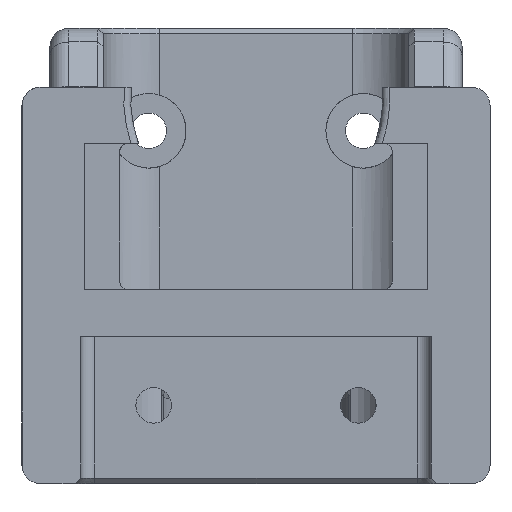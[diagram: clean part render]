
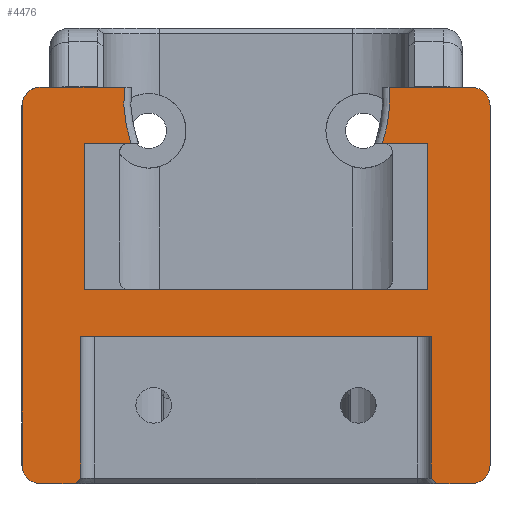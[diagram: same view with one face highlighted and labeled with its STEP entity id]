
A CAD part, front view. The second image highlights one B-rep face of the part: STEP entity #4476.
In plain terms, the highlighted planar face has unit normal (0, -1, 0).
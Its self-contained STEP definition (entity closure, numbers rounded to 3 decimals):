
#76=ELLIPSE('',#4882,2.,2.);
#77=ELLIPSE('',#4885,2.,2.);
#150=PLANE('',#4881);
#224=LINE('',#6659,#567);
#228=LINE('',#6671,#571);
#399=LINE('',#8443,#742);
#424=LINE('',#8539,#767);
#440=LINE('',#8845,#783);
#442=LINE('',#8940,#785);
#446=LINE('',#8950,#789);
#447=LINE('',#8953,#790);
#448=LINE('',#8955,#791);
#449=LINE('',#8957,#792);
#450=LINE('',#8959,#793);
#451=LINE('',#8960,#794);
#452=LINE('',#8964,#795);
#453=LINE('',#8968,#796);
#454=LINE('',#8970,#797);
#455=LINE('',#8971,#798);
#567=VECTOR('',#5177,10.);
#571=VECTOR('',#5185,10.);
#742=VECTOR('',#5724,10.);
#767=VECTOR('',#5797,10.);
#783=VECTOR('',#5869,10.);
#785=VECTOR('',#5881,10.);
#789=VECTOR('',#5889,10.);
#790=VECTOR('',#5892,10.);
#791=VECTOR('',#5893,10.);
#792=VECTOR('',#5894,10.);
#793=VECTOR('',#5895,10.);
#794=VECTOR('',#5896,10.);
#795=VECTOR('',#5899,10.);
#796=VECTOR('',#5904,10.);
#797=VECTOR('',#5905,10.);
#798=VECTOR('',#5906,10.);
#1164=FACE_OUTER_BOUND('',#1435,.T.);
#1435=EDGE_LOOP('',(#3844,#3845,#3846,#3847,#3848,#3849,#3850,#3851,#3852,
#3853,#3854,#3855,#3856,#3857,#3858,#3859,#3860,#3861,#3862,#3863,#3864,
#3865));
#1669=CIRCLE('',#4879,14.25);
#1670=CIRCLE('',#4883,2.);
#1671=CIRCLE('',#4884,2.);
#1672=CIRCLE('',#4886,14.25);
#1892=VERTEX_POINT('',#6656);
#1893=VERTEX_POINT('',#6658);
#1898=VERTEX_POINT('',#6668);
#1899=VERTEX_POINT('',#6670);
#2113=VERTEX_POINT('',#8440);
#2114=VERTEX_POINT('',#8442);
#2134=VERTEX_POINT('',#8527);
#2135=VERTEX_POINT('',#8538);
#2167=VERTEX_POINT('',#8842);
#2168=VERTEX_POINT('',#8844);
#2171=VERTEX_POINT('',#8926);
#2172=VERTEX_POINT('',#8939);
#2175=VERTEX_POINT('',#8947);
#2176=VERTEX_POINT('',#8949);
#2177=VERTEX_POINT('',#8952);
#2178=VERTEX_POINT('',#8954);
#2179=VERTEX_POINT('',#8956);
#2180=VERTEX_POINT('',#8958);
#2181=VERTEX_POINT('',#8961);
#2182=VERTEX_POINT('',#8963);
#2183=VERTEX_POINT('',#8967);
#2184=VERTEX_POINT('',#8969);
#2329=EDGE_CURVE('',#1892,#1893,#224,.T.);
#2335=EDGE_CURVE('',#1898,#1899,#228,.T.);
#2673=EDGE_CURVE('',#2114,#2113,#399,.T.);
#2710=EDGE_CURVE('',#2134,#2135,#424,.T.);
#2757=EDGE_CURVE('',#2167,#2168,#440,.T.);
#2763=EDGE_CURVE('',#2114,#2171,#1669,.T.);
#2765=EDGE_CURVE('',#2171,#2172,#442,.T.);
#2769=EDGE_CURVE('',#2175,#2113,#76,.T.);
#2770=EDGE_CURVE('',#2176,#2175,#446,.T.);
#2771=EDGE_CURVE('',#1899,#2176,#1670,.T.);
#2772=EDGE_CURVE('',#2177,#1898,#447,.T.);
#2773=EDGE_CURVE('',#2177,#2178,#448,.T.);
#2774=EDGE_CURVE('',#2178,#2179,#449,.T.);
#2775=EDGE_CURVE('',#2180,#2179,#450,.T.);
#2776=EDGE_CURVE('',#1893,#2180,#451,.T.);
#2777=EDGE_CURVE('',#2181,#1892,#1671,.T.);
#2778=EDGE_CURVE('',#2181,#2182,#452,.T.);
#2779=EDGE_CURVE('',#2135,#2182,#77,.T.);
#2780=EDGE_CURVE('',#2168,#2134,#1672,.T.);
#2781=EDGE_CURVE('',#2167,#2183,#453,.T.);
#2782=EDGE_CURVE('',#2183,#2184,#454,.T.);
#2783=EDGE_CURVE('',#2184,#2172,#455,.T.);
#3844=ORIENTED_EDGE('',*,*,#2763,.F.);
#3845=ORIENTED_EDGE('',*,*,#2673,.T.);
#3846=ORIENTED_EDGE('',*,*,#2769,.F.);
#3847=ORIENTED_EDGE('',*,*,#2770,.F.);
#3848=ORIENTED_EDGE('',*,*,#2771,.F.);
#3849=ORIENTED_EDGE('',*,*,#2335,.F.);
#3850=ORIENTED_EDGE('',*,*,#2772,.F.);
#3851=ORIENTED_EDGE('',*,*,#2773,.T.);
#3852=ORIENTED_EDGE('',*,*,#2774,.T.);
#3853=ORIENTED_EDGE('',*,*,#2775,.F.);
#3854=ORIENTED_EDGE('',*,*,#2776,.F.);
#3855=ORIENTED_EDGE('',*,*,#2329,.F.);
#3856=ORIENTED_EDGE('',*,*,#2777,.F.);
#3857=ORIENTED_EDGE('',*,*,#2778,.T.);
#3858=ORIENTED_EDGE('',*,*,#2779,.F.);
#3859=ORIENTED_EDGE('',*,*,#2710,.F.);
#3860=ORIENTED_EDGE('',*,*,#2780,.F.);
#3861=ORIENTED_EDGE('',*,*,#2757,.F.);
#3862=ORIENTED_EDGE('',*,*,#2781,.T.);
#3863=ORIENTED_EDGE('',*,*,#2782,.T.);
#3864=ORIENTED_EDGE('',*,*,#2783,.T.);
#3865=ORIENTED_EDGE('',*,*,#2765,.F.);
#4476=ADVANCED_FACE('',(#1164),#150,.T.);
#4879=AXIS2_PLACEMENT_3D('',#8927,#5877,#5878);
#4881=AXIS2_PLACEMENT_3D('',#8946,#5885,#5886);
#4882=AXIS2_PLACEMENT_3D('',#8948,#5887,#5888);
#4883=AXIS2_PLACEMENT_3D('',#8951,#5890,#5891);
#4884=AXIS2_PLACEMENT_3D('',#8962,#5897,#5898);
#4885=AXIS2_PLACEMENT_3D('',#8965,#5900,#5901);
#4886=AXIS2_PLACEMENT_3D('',#8966,#5902,#5903);
#5177=DIRECTION('',(-1.,0.,0.));
#5185=DIRECTION('',(-1.,0.,0.));
#5724=DIRECTION('',(-1.,0.,0.));
#5797=DIRECTION('',(1.,0.,0.));
#5869=DIRECTION('',(-1.,0.,0.));
#5877=DIRECTION('center_axis',(0.,-1.,0.));
#5878=DIRECTION('ref_axis',(-0.992,0.,-0.127));
#5881=DIRECTION('',(-1.,0.,0.));
#5885=DIRECTION('center_axis',(0.,-1.,0.));
#5886=DIRECTION('ref_axis',(1.,0.,0.));
#5887=DIRECTION('center_axis',(0.,1.,0.));
#5888=DIRECTION('ref_axis',(0.,0.,1.));
#5889=DIRECTION('',(0.,0.,1.));
#5890=DIRECTION('center_axis',(0.,1.,0.));
#5891=DIRECTION('ref_axis',(-0.707,0.,-0.707));
#5892=DIRECTION('',(-0.707,0.,-0.707));
#5893=DIRECTION('',(0.,0.,1.));
#5894=DIRECTION('',(1.,0.,0.));
#5895=DIRECTION('',(0.,0.,1.));
#5896=DIRECTION('',(-0.707,0.,0.707));
#5897=DIRECTION('center_axis',(0.,1.,0.));
#5898=DIRECTION('ref_axis',(0.707,0.,-0.707));
#5899=DIRECTION('',(0.,0.,1.));
#5900=DIRECTION('center_axis',(0.,1.,0.));
#5901=DIRECTION('ref_axis',(0.,0.,1.));
#5902=DIRECTION('center_axis',(0.,-1.,0.));
#5903=DIRECTION('ref_axis',(0.992,0.,-0.127));
#5904=DIRECTION('',(0.,0.,-1.));
#5905=DIRECTION('',(-1.,0.,0.));
#5906=DIRECTION('',(0.,0.,1.));
#6656=CARTESIAN_POINT('',(39.053,-26.,-157.388));
#6658=CARTESIAN_POINT('',(35.353,-26.,-157.388));
#6659=CARTESIAN_POINT('',(26.915,-26.,-157.388));
#6668=CARTESIAN_POINT('',(-3.4,-26.,-157.388));
#6670=CARTESIAN_POINT('',(-7.1,-26.,-157.388));
#6671=CARTESIAN_POINT('',(26.915,-26.,-157.388));
#8440=CARTESIAN_POINT('',(-7.1,-26.,-114.899));
#8442=CARTESIAN_POINT('',(1.865,-26.,-114.899));
#8443=CARTESIAN_POINT('',(-5.325,-26.,-114.899));
#8527=CARTESIAN_POINT('',(30.24,-26.,-114.899));
#8538=CARTESIAN_POINT('',(39.053,-26.,-114.899));
#8539=CARTESIAN_POINT('',(37.278,-26.,-114.899));
#8842=CARTESIAN_POINT('',(34.353,-26.,-120.899));
#8844=CARTESIAN_POINT('',(29.517,-26.,-120.899));
#8845=CARTESIAN_POINT('',(26.84,-26.,-120.899));
#8926=CARTESIAN_POINT('',(2.588,-26.,-120.899));
#8927=CARTESIAN_POINT('Origin',(16.053,-26.,-116.233));
#8939=CARTESIAN_POINT('',(-2.4,-26.,-120.899));
#8940=CARTESIAN_POINT('',(26.84,-26.,-120.899));
#8946=CARTESIAN_POINT('Origin',(-5.9,-26.,-136.589));
#8947=CARTESIAN_POINT('',(-9.1,-26.,-116.899));
#8948=CARTESIAN_POINT('Origin',(-7.1,-26.,-116.899));
#8949=CARTESIAN_POINT('',(-9.1,-26.,-155.388));
#8950=CARTESIAN_POINT('',(-9.1,-26.,-157.388));
#8951=CARTESIAN_POINT('Origin',(-7.1,-26.,-155.388));
#8952=CARTESIAN_POINT('',(-2.8,-26.,-156.788));
#8953=CARTESIAN_POINT('',(1.325,-26.,-152.663));
#8954=CARTESIAN_POINT('',(-2.8,-26.,-141.588));
#8955=CARTESIAN_POINT('',(-2.8,-26.,-143.888));
#8956=CARTESIAN_POINT('',(34.753,-26.,-141.588));
#8957=CARTESIAN_POINT('',(-4.5,-26.,-141.589));
#8958=CARTESIAN_POINT('',(34.753,-26.,-156.788));
#8959=CARTESIAN_POINT('',(34.753,-26.,-151.488));
#8960=CARTESIAN_POINT('',(19.69,-26.,-141.725));
#8961=CARTESIAN_POINT('',(41.053,-26.,-155.388));
#8962=CARTESIAN_POINT('Origin',(39.053,-26.,-155.388));
#8963=CARTESIAN_POINT('',(41.053,-26.,-116.899));
#8964=CARTESIAN_POINT('',(41.053,-26.,-157.388));
#8965=CARTESIAN_POINT('Origin',(39.053,-26.,-116.899));
#8966=CARTESIAN_POINT('Origin',(16.053,-26.,-116.233));
#8967=CARTESIAN_POINT('',(34.353,-26.,-136.589));
#8968=CARTESIAN_POINT('',(34.353,-26.,-125.744));
#8969=CARTESIAN_POINT('',(-2.4,-26.,-136.589));
#8970=CARTESIAN_POINT('',(-3.15,-26.,-136.589));
#8971=CARTESIAN_POINT('',(-2.4,-26.,-136.589));
